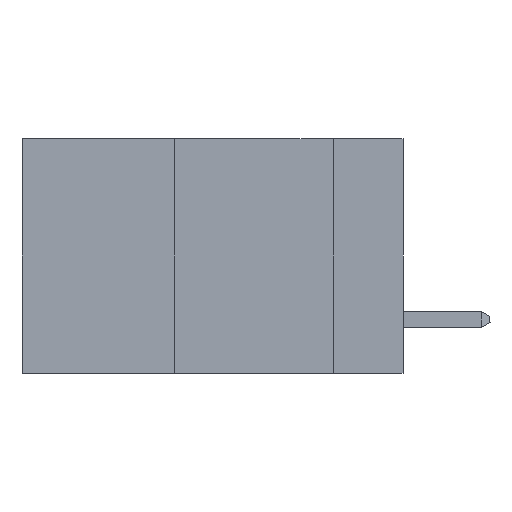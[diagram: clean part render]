
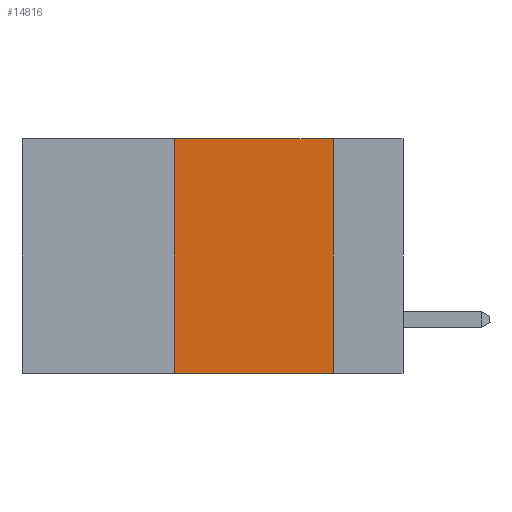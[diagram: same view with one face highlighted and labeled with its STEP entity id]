
A CAD part, left-side view. The second image highlights one B-rep face of the part: STEP entity #14816.
In plain terms, the highlighted planar face has unit normal (-1, 0, 0).
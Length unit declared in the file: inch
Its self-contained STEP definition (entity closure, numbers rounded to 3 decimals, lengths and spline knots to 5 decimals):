
#58 = LINE ( 'NONE', #7962, #6805 ) ;
#776 = DIRECTION ( 'NONE',  ( 1., 0., 0. ) ) ;
#904 = EDGE_CURVE ( 'NONE', #3700, #13778, #15842, .T. ) ;
#1277 = ORIENTED_EDGE ( 'NONE', *, *, #904, .F. ) ;
#2782 = CARTESIAN_POINT ( 'NONE',  ( 0., 0.6, -0.37 ) ) ;
#3151 = DIRECTION ( 'NONE',  ( 0., 0., 1. ) ) ;
#3700 = VERTEX_POINT ( 'NONE', #17175 ) ;
#4275 = CARTESIAN_POINT ( 'NONE',  ( 0., 0.6, 0. ) ) ;
#4468 = DIRECTION ( 'NONE',  ( 0., -1., 0. ) ) ;
#4696 = VECTOR ( 'NONE', #17999, 39.37008 ) ;
#4906 = EDGE_LOOP ( 'NONE', ( #1277, #7905, #17274, #16611 ) ) ;
#5173 = CARTESIAN_POINT ( 'NONE',  ( 0., 0.6, 0. ) ) ;
#6380 = VERTEX_POINT ( 'NONE', #22107 ) ;
#6805 = VECTOR ( 'NONE', #3151, 39.37008 ) ;
#7905 = ORIENTED_EDGE ( 'NONE', *, *, #16748, .F. ) ;
#7962 = CARTESIAN_POINT ( 'NONE',  ( 0., 0.36, 0. ) ) ;
#8568 = VECTOR ( 'NONE', #21040, 39.37008 ) ;
#8916 = CARTESIAN_POINT ( 'NONE',  ( 0., 0.11, 0. ) ) ;
#9558 = DIRECTION ( 'NONE',  ( 0., 0., -1. ) ) ;
#11010 = PLANE ( 'NONE',  #12461 ) ;
#11899 = CARTESIAN_POINT ( 'NONE',  ( 0., 0.36, 0. ) ) ;
#12207 = EDGE_CURVE ( 'NONE', #6380, #19084, #58, .T. ) ;
#12461 = AXIS2_PLACEMENT_3D ( 'NONE', #4275, #776, #9558 ) ;
#13173 = LINE ( 'NONE', #5173, #8568 ) ;
#13236 = LINE ( 'NONE', #2782, #20289 ) ;
#13778 = VERTEX_POINT ( 'NONE', #18190 ) ;
#14816 = ADVANCED_FACE ( 'NONE', ( #16217 ), #11010, .F. ) ;
#15842 = LINE ( 'NONE', #8916, #4696 ) ;
#16217 = FACE_OUTER_BOUND ( 'NONE', #4906, .T. ) ;
#16611 = ORIENTED_EDGE ( 'NONE', *, *, #20245, .T. ) ;
#16748 = EDGE_CURVE ( 'NONE', #19084, #3700, #13173, .T. ) ;
#17175 = CARTESIAN_POINT ( 'NONE',  ( 0., 0.11, 0. ) ) ;
#17274 = ORIENTED_EDGE ( 'NONE', *, *, #12207, .F. ) ;
#17999 = DIRECTION ( 'NONE',  ( 0., 0., -1. ) ) ;
#18190 = CARTESIAN_POINT ( 'NONE',  ( 0., 0.11, -0.37 ) ) ;
#19084 = VERTEX_POINT ( 'NONE', #11899 ) ;
#20245 = EDGE_CURVE ( 'NONE', #6380, #13778, #13236, .T. ) ;
#20289 = VECTOR ( 'NONE', #4468, 39.37008 ) ;
#21040 = DIRECTION ( 'NONE',  ( 0., -1., 0. ) ) ;
#22107 = CARTESIAN_POINT ( 'NONE',  ( 0., 0.36, -0.37 ) ) ;
